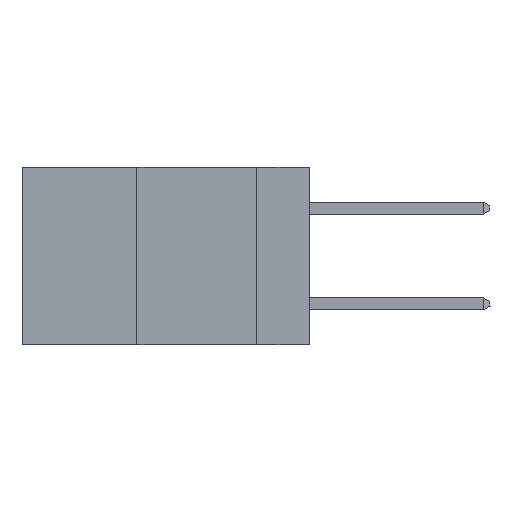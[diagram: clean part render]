
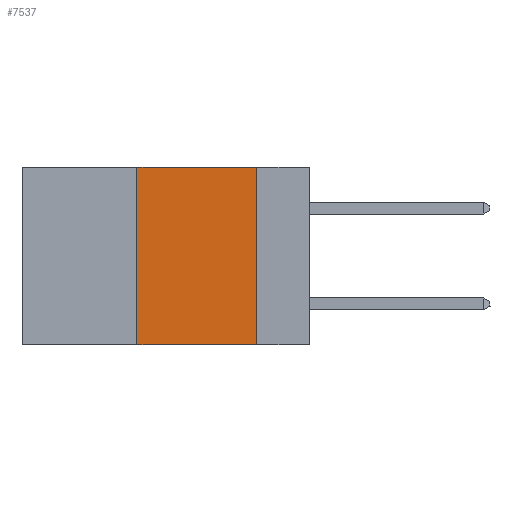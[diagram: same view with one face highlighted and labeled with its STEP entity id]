
A CAD part, left-side view. The second image highlights one B-rep face of the part: STEP entity #7537.
In plain terms, the highlighted planar face has unit normal (-1, 0, 0).
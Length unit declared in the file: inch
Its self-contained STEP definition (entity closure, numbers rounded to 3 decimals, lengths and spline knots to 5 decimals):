
#303 = CARTESIAN_POINT ( 'NONE',  ( 0., 0.6, -0.37 ) ) ;
#327 = DIRECTION ( 'NONE',  ( 0., 0., -1. ) ) ;
#599 = VECTOR ( 'NONE', #7029, 39.37008 ) ;
#679 = LINE ( 'NONE', #303, #5998 ) ;
#1361 = CARTESIAN_POINT ( 'NONE',  ( 0., 0.11, -0.37 ) ) ;
#1919 = VERTEX_POINT ( 'NONE', #6002 ) ;
#2214 = LINE ( 'NONE', #8706, #4198 ) ;
#2660 = PLANE ( 'NONE',  #5072 ) ;
#2723 = VERTEX_POINT ( 'NONE', #4624 ) ;
#3098 = FACE_OUTER_BOUND ( 'NONE', #5768, .T. ) ;
#3104 = ORIENTED_EDGE ( 'NONE', *, *, #9716, .F. ) ;
#3273 = VERTEX_POINT ( 'NONE', #7841 ) ;
#3458 = ORIENTED_EDGE ( 'NONE', *, *, #6860, .T. ) ;
#3486 = CARTESIAN_POINT ( 'NONE',  ( 0., 0.6, 0. ) ) ;
#4198 = VECTOR ( 'NONE', #7986, 39.37008 ) ;
#4624 = CARTESIAN_POINT ( 'NONE',  ( 0., 0.11, 0. ) ) ;
#5072 = AXIS2_PLACEMENT_3D ( 'NONE', #3486, #8296, #327 ) ;
#5505 = VERTEX_POINT ( 'NONE', #1361 ) ;
#5768 = EDGE_LOOP ( 'NONE', ( #3104, #8109, #9177, #3458 ) ) ;
#5837 = DIRECTION ( 'NONE',  ( 0., -1., 0. ) ) ;
#5962 = CARTESIAN_POINT ( 'NONE',  ( 0., 0.6, 0. ) ) ;
#5998 = VECTOR ( 'NONE', #5837, 39.37008 ) ;
#6002 = CARTESIAN_POINT ( 'NONE',  ( 0., 0.36, -0.37 ) ) ;
#6046 = LINE ( 'NONE', #10168, #599 ) ;
#6847 = LINE ( 'NONE', #5962, #7839 ) ;
#6860 = EDGE_CURVE ( 'NONE', #1919, #5505, #679, .T. ) ;
#6877 = DIRECTION ( 'NONE',  ( 0., -1., 0. ) ) ;
#7029 = DIRECTION ( 'NONE',  ( 0., 0., -1. ) ) ;
#7537 = ADVANCED_FACE ( 'NONE', ( #3098 ), #2660, .F. ) ;
#7730 = EDGE_CURVE ( 'NONE', #3273, #2723, #6847, .T. ) ;
#7839 = VECTOR ( 'NONE', #6877, 39.37008 ) ;
#7841 = CARTESIAN_POINT ( 'NONE',  ( 0., 0.36, 0. ) ) ;
#7986 = DIRECTION ( 'NONE',  ( 0., 0., 1. ) ) ;
#8109 = ORIENTED_EDGE ( 'NONE', *, *, #7730, .F. ) ;
#8296 = DIRECTION ( 'NONE',  ( 1., 0., 0. ) ) ;
#8405 = EDGE_CURVE ( 'NONE', #1919, #3273, #2214, .T. ) ;
#8706 = CARTESIAN_POINT ( 'NONE',  ( 0., 0.36, 0. ) ) ;
#9177 = ORIENTED_EDGE ( 'NONE', *, *, #8405, .F. ) ;
#9716 = EDGE_CURVE ( 'NONE', #2723, #5505, #6046, .T. ) ;
#10168 = CARTESIAN_POINT ( 'NONE',  ( 0., 0.11, 0. ) ) ;
